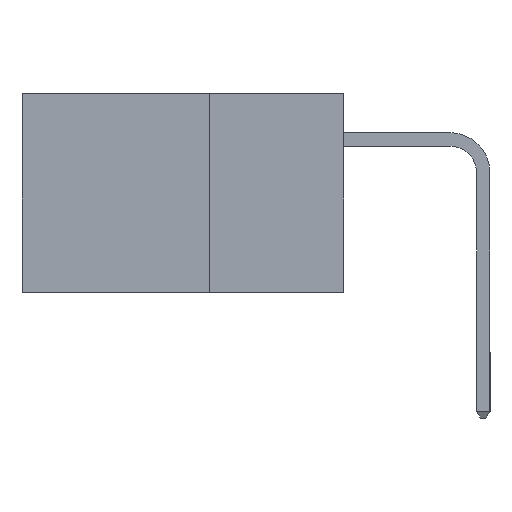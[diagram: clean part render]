
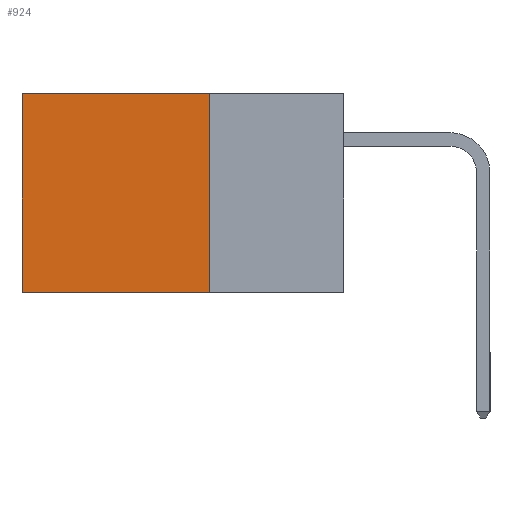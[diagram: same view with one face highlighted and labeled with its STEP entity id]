
A CAD part, left-side view. The second image highlights one B-rep face of the part: STEP entity #924.
In plain terms, the highlighted planar face has unit normal (-1, 0, 0).
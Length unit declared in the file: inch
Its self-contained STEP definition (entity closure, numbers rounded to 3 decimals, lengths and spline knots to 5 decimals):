
#189 = EDGE_CURVE ( 'NONE', #17737, #12247, #7020, .T. ) ;
#313 = DIRECTION ( 'NONE',  ( 0., 1., 0. ) ) ;
#906 = DIRECTION ( 'NONE',  ( 1., 0., 0. ) ) ;
#924 = ADVANCED_FACE ( 'NONE', ( #10123 ), #13689, .F. ) ;
#1202 = ORIENTED_EDGE ( 'NONE', *, *, #15032, .F. ) ;
#1472 = LINE ( 'NONE', #17163, #10181 ) ;
#1672 = DIRECTION ( 'NONE',  ( 0., 0., -1. ) ) ;
#2627 = LINE ( 'NONE', #9073, #10439 ) ;
#3226 = EDGE_CURVE ( 'NONE', #17737, #14612, #2627, .T. ) ;
#4924 = LINE ( 'NONE', #11655, #15142 ) ;
#6194 = ORIENTED_EDGE ( 'NONE', *, *, #189, .T. ) ;
#7020 = LINE ( 'NONE', #14545, #14124 ) ;
#8036 = CARTESIAN_POINT ( 'NONE',  ( 0.298, 0.6, 0. ) ) ;
#8053 = AXIS2_PLACEMENT_3D ( 'NONE', #13516, #906, #16361 ) ;
#9073 = CARTESIAN_POINT ( 'NONE',  ( 0.298, 0.25, 0. ) ) ;
#9403 = VERTEX_POINT ( 'NONE', #15754 ) ;
#9737 = ORIENTED_EDGE ( 'NONE', *, *, #3226, .F. ) ;
#10123 = FACE_OUTER_BOUND ( 'NONE', #13726, .T. ) ;
#10181 = VECTOR ( 'NONE', #313, 39.37008 ) ;
#10416 = DIRECTION ( 'NONE',  ( 0., 1., 0. ) ) ;
#10439 = VECTOR ( 'NONE', #10500, 39.37008 ) ;
#10500 = DIRECTION ( 'NONE',  ( 0., 0., -1. ) ) ;
#11655 = CARTESIAN_POINT ( 'NONE',  ( 0.298, 0.6, 0. ) ) ;
#12247 = VERTEX_POINT ( 'NONE', #8036 ) ;
#12304 = EDGE_CURVE ( 'NONE', #12247, #9403, #4924, .T. ) ;
#12316 = ORIENTED_EDGE ( 'NONE', *, *, #12304, .T. ) ;
#12961 = CARTESIAN_POINT ( 'NONE',  ( 0.298, 0.25, 0. ) ) ;
#13516 = CARTESIAN_POINT ( 'NONE',  ( 0.298, 0.25, 0. ) ) ;
#13689 = PLANE ( 'NONE',  #8053 ) ;
#13701 = CARTESIAN_POINT ( 'NONE',  ( 0.298, 0.25, -0.37 ) ) ;
#13726 = EDGE_LOOP ( 'NONE', ( #12316, #1202, #9737, #6194 ) ) ;
#14124 = VECTOR ( 'NONE', #10416, 39.37008 ) ;
#14545 = CARTESIAN_POINT ( 'NONE',  ( 0.298, 0.25, 0. ) ) ;
#14612 = VERTEX_POINT ( 'NONE', #13701 ) ;
#15032 = EDGE_CURVE ( 'NONE', #14612, #9403, #1472, .T. ) ;
#15142 = VECTOR ( 'NONE', #1672, 39.37008 ) ;
#15754 = CARTESIAN_POINT ( 'NONE',  ( 0.298, 0.6, -0.37 ) ) ;
#16361 = DIRECTION ( 'NONE',  ( 0., 0., -1. ) ) ;
#17163 = CARTESIAN_POINT ( 'NONE',  ( 0.298, 0.25, -0.37 ) ) ;
#17737 = VERTEX_POINT ( 'NONE', #12961 ) ;
